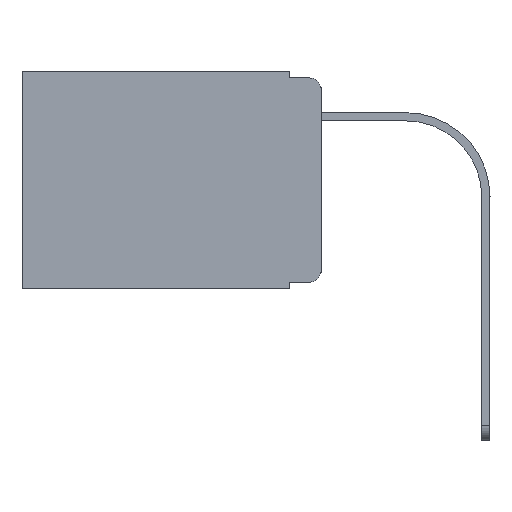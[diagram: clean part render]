
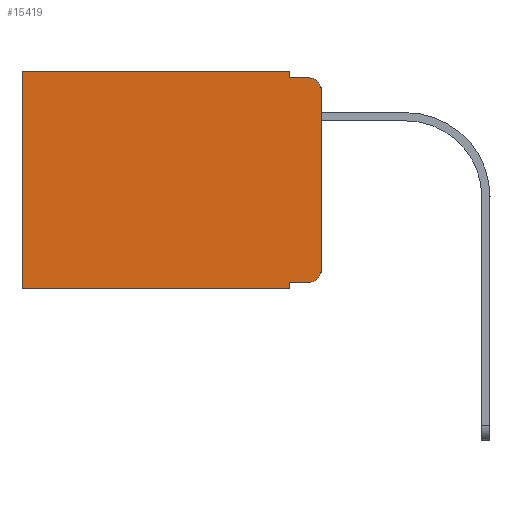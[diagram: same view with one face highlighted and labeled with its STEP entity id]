
A CAD part, left-side view. The second image highlights one B-rep face of the part: STEP entity #15419.
In plain terms, the highlighted planar face has unit normal (-1, 0, 0).
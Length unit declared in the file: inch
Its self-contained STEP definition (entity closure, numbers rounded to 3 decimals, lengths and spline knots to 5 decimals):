
#415 = DIRECTION ( 'NONE',  ( 0., 1., 0. ) ) ;
#570 = CARTESIAN_POINT ( 'NONE',  ( 0.298, 0.02, -0.313 ) ) ;
#605 = VERTEX_POINT ( 'NONE', #16347 ) ;
#705 = VECTOR ( 'NONE', #16839, 39.37008 ) ;
#754 = EDGE_CURVE ( 'NONE', #12853, #17186, #12519, .T. ) ;
#1457 = AXIS2_PLACEMENT_3D ( 'NONE', #570, #11318, #12686 ) ;
#1466 = LINE ( 'NONE', #13825, #13995 ) ;
#1472 = DIRECTION ( 'NONE',  ( 0., 0., -1. ) ) ;
#1633 = LINE ( 'NONE', #10139, #11518 ) ;
#1658 = DIRECTION ( 'NONE',  ( 0., 0., -1. ) ) ;
#2054 = LINE ( 'NONE', #6302, #6958 ) ;
#2212 = VERTEX_POINT ( 'NONE', #8740 ) ;
#2219 = LINE ( 'NONE', #16582, #17945 ) ;
#2535 = AXIS2_PLACEMENT_3D ( 'NONE', #10238, #14729, #13340 ) ;
#2825 = ORIENTED_EDGE ( 'NONE', *, *, #10671, .F. ) ;
#2854 = CARTESIAN_POINT ( 'NONE',  ( 0.298, 0., 0. ) ) ;
#3688 = CARTESIAN_POINT ( 'NONE',  ( 0.298, 0.02, -0.01 ) ) ;
#3974 = DIRECTION ( 'NONE',  ( 0., -1., 0. ) ) ;
#4005 = CARTESIAN_POINT ( 'NONE',  ( 0.298, 0.051, -0.01 ) ) ;
#4015 = CARTESIAN_POINT ( 'NONE',  ( 0.298, 0., -0.313 ) ) ;
#4372 = LINE ( 'NONE', #9723, #4974 ) ;
#4430 = CARTESIAN_POINT ( 'NONE',  ( 0.298, 0., -0.343 ) ) ;
#4444 = VECTOR ( 'NONE', #1658, 39.37008 ) ;
#4490 = CARTESIAN_POINT ( 'NONE',  ( 0.298, 0.473, 0. ) ) ;
#4757 = EDGE_CURVE ( 'NONE', #6436, #8206, #2219, .T. ) ;
#4974 = VECTOR ( 'NONE', #9996, 39.37008 ) ;
#5098 = DIRECTION ( 'NONE',  ( 0., -1., 0. ) ) ;
#5532 = DIRECTION ( 'NONE',  ( 0., 0., -1. ) ) ;
#5860 = ORIENTED_EDGE ( 'NONE', *, *, #15151, .T. ) ;
#6302 = CARTESIAN_POINT ( 'NONE',  ( 0.298, 0.051, 0. ) ) ;
#6436 = VERTEX_POINT ( 'NONE', #8310 ) ;
#6469 = CIRCLE ( 'NONE', #1457, 0.02 ) ;
#6568 = EDGE_CURVE ( 'NONE', #605, #14720, #1466, .T. ) ;
#6696 = ORIENTED_EDGE ( 'NONE', *, *, #754, .F. ) ;
#6855 = ORIENTED_EDGE ( 'NONE', *, *, #15969, .T. ) ;
#6892 = VERTEX_POINT ( 'NONE', #9403 ) ;
#6958 = VECTOR ( 'NONE', #11914, 39.37008 ) ;
#7085 = LINE ( 'NONE', #4430, #705 ) ;
#7919 = CARTESIAN_POINT ( 'NONE',  ( 0.298, 0.02, -0.333 ) ) ;
#8130 = CIRCLE ( 'NONE', #2535, 0.02 ) ;
#8206 = VERTEX_POINT ( 'NONE', #7919 ) ;
#8284 = VERTEX_POINT ( 'NONE', #9853 ) ;
#8310 = CARTESIAN_POINT ( 'NONE',  ( 0.298, 0.051, -0.333 ) ) ;
#8314 = DIRECTION ( 'NONE',  ( 1., 0., 0. ) ) ;
#8740 = CARTESIAN_POINT ( 'NONE',  ( 0.298, 0.051, -0.343 ) ) ;
#8786 = ORIENTED_EDGE ( 'NONE', *, *, #18202, .F. ) ;
#9403 = CARTESIAN_POINT ( 'NONE',  ( 0.298, 0.473, -0.343 ) ) ;
#9607 = PLANE ( 'NONE',  #9995 ) ;
#9723 = CARTESIAN_POINT ( 'NONE',  ( 0.298, 0.473, 0. ) ) ;
#9853 = CARTESIAN_POINT ( 'NONE',  ( 0.298, 0.051, 0. ) ) ;
#9985 = EDGE_LOOP ( 'NONE', ( #13382, #10101, #6696, #8786, #12855, #5860, #2825, #14494, #11599, #6855 ) ) ;
#9995 = AXIS2_PLACEMENT_3D ( 'NONE', #2854, #8314, #1472 ) ;
#9996 = DIRECTION ( 'NONE',  ( 0., 0., -1. ) ) ;
#10101 = ORIENTED_EDGE ( 'NONE', *, *, #12127, .T. ) ;
#10139 = CARTESIAN_POINT ( 'NONE',  ( 0.298, 0., 0. ) ) ;
#10238 = CARTESIAN_POINT ( 'NONE',  ( 0.298, 0.02, -0.03 ) ) ;
#10671 = EDGE_CURVE ( 'NONE', #2212, #6892, #7085, .T. ) ;
#11318 = DIRECTION ( 'NONE',  ( -1., 0., 0. ) ) ;
#11518 = VECTOR ( 'NONE', #415, 39.37008 ) ;
#11599 = ORIENTED_EDGE ( 'NONE', *, *, #4757, .T. ) ;
#11914 = DIRECTION ( 'NONE',  ( 0., 0., -1. ) ) ;
#12127 = EDGE_CURVE ( 'NONE', #605, #17186, #8130, .T. ) ;
#12519 = LINE ( 'NONE', #16588, #16215 ) ;
#12686 = DIRECTION ( 'NONE',  ( 0., 0., -1. ) ) ;
#12853 = VERTEX_POINT ( 'NONE', #4005 ) ;
#12855 = ORIENTED_EDGE ( 'NONE', *, *, #17505, .T. ) ;
#13093 = EDGE_CURVE ( 'NONE', #6436, #2212, #2054, .T. ) ;
#13340 = DIRECTION ( 'NONE',  ( 0., 0., -1. ) ) ;
#13382 = ORIENTED_EDGE ( 'NONE', *, *, #6568, .F. ) ;
#13825 = CARTESIAN_POINT ( 'NONE',  ( 0.298, 0., 0. ) ) ;
#13995 = VECTOR ( 'NONE', #5532, 39.37008 ) ;
#14274 = CARTESIAN_POINT ( 'NONE',  ( 0.298, 0.051, 0. ) ) ;
#14494 = ORIENTED_EDGE ( 'NONE', *, *, #13093, .F. ) ;
#14720 = VERTEX_POINT ( 'NONE', #4015 ) ;
#14729 = DIRECTION ( 'NONE',  ( -1., 0., 0. ) ) ;
#15151 = EDGE_CURVE ( 'NONE', #17894, #6892, #4372, .T. ) ;
#15419 = ADVANCED_FACE ( 'NONE', ( #18048 ), #9607, .F. ) ;
#15555 = LINE ( 'NONE', #14274, #4444 ) ;
#15969 = EDGE_CURVE ( 'NONE', #8206, #14720, #6469, .T. ) ;
#16215 = VECTOR ( 'NONE', #5098, 39.37008 ) ;
#16347 = CARTESIAN_POINT ( 'NONE',  ( 0.298, 0., -0.03 ) ) ;
#16582 = CARTESIAN_POINT ( 'NONE',  ( 0.298, 0.051, -0.333 ) ) ;
#16588 = CARTESIAN_POINT ( 'NONE',  ( 0.298, 0.051, -0.01 ) ) ;
#16839 = DIRECTION ( 'NONE',  ( 0., 1., 0. ) ) ;
#17186 = VERTEX_POINT ( 'NONE', #3688 ) ;
#17505 = EDGE_CURVE ( 'NONE', #8284, #17894, #1633, .T. ) ;
#17894 = VERTEX_POINT ( 'NONE', #4490 ) ;
#17945 = VECTOR ( 'NONE', #3974, 39.37008 ) ;
#18048 = FACE_OUTER_BOUND ( 'NONE', #9985, .T. ) ;
#18202 = EDGE_CURVE ( 'NONE', #8284, #12853, #15555, .T. ) ;
